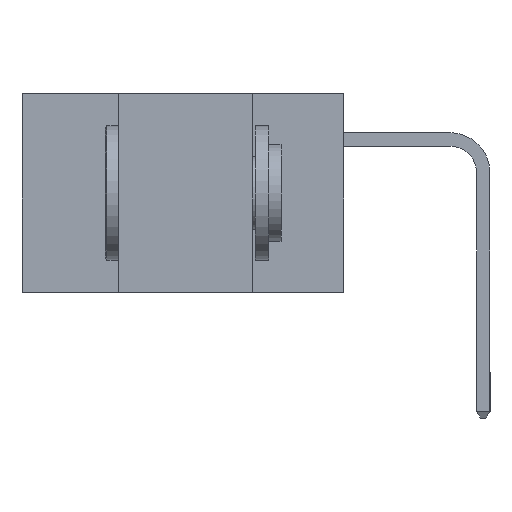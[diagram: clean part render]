
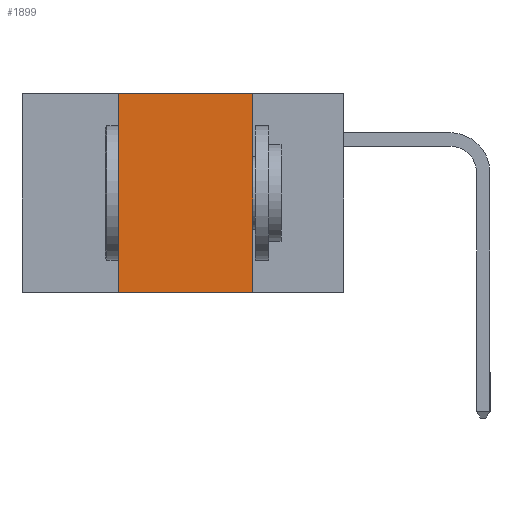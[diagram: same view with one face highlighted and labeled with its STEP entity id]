
A CAD part, left-side view. The second image highlights one B-rep face of the part: STEP entity #1899.
In plain terms, the highlighted planar face has unit normal (-1, 0, 0).
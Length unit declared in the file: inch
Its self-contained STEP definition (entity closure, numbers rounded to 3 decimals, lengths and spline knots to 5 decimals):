
#573 = LINE ( 'NONE', #4851, #6733 ) ;
#735 = CARTESIAN_POINT ( 'NONE',  ( 0., 0.42, 0. ) ) ;
#907 = DIRECTION ( 'NONE',  ( 0., -1., 0. ) ) ;
#1231 = CARTESIAN_POINT ( 'NONE',  ( 0., 0.17, -0.37 ) ) ;
#1440 = CARTESIAN_POINT ( 'NONE',  ( 0., 0.17, 0. ) ) ;
#1478 = LINE ( 'NONE', #7934, #7144 ) ;
#1799 = DIRECTION ( 'NONE',  ( 0., -1., 0. ) ) ;
#1844 = FACE_OUTER_BOUND ( 'NONE', #6764, .T. ) ;
#1899 = ADVANCED_FACE ( 'NONE', ( #1844 ), #7327, .F. ) ;
#2058 = AXIS2_PLACEMENT_3D ( 'NONE', #9640, #7390, #8138 ) ;
#2682 = EDGE_CURVE ( 'NONE', #4885, #6575, #4917, .T. ) ;
#3073 = ORIENTED_EDGE ( 'NONE', *, *, #7440, .F. ) ;
#3139 = VECTOR ( 'NONE', #6104, 39.37008 ) ;
#3254 = DIRECTION ( 'NONE',  ( 0., 0., 1. ) ) ;
#3515 = EDGE_CURVE ( 'NONE', #7877, #6575, #573, .T. ) ;
#4851 = CARTESIAN_POINT ( 'NONE',  ( 0., 0.6, -0.37 ) ) ;
#4885 = VERTEX_POINT ( 'NONE', #5595 ) ;
#4917 = LINE ( 'NONE', #1440, #3139 ) ;
#5148 = ORIENTED_EDGE ( 'NONE', *, *, #7636, .F. ) ;
#5404 = LINE ( 'NONE', #8667, #6499 ) ;
#5595 = CARTESIAN_POINT ( 'NONE',  ( 0., 0.17, 0. ) ) ;
#6104 = DIRECTION ( 'NONE',  ( 0., 0., -1. ) ) ;
#6499 = VECTOR ( 'NONE', #907, 39.37008 ) ;
#6575 = VERTEX_POINT ( 'NONE', #1231 ) ;
#6733 = VECTOR ( 'NONE', #1799, 39.37008 ) ;
#6764 = EDGE_LOOP ( 'NONE', ( #8663, #5148, #3073, #9223 ) ) ;
#7144 = VECTOR ( 'NONE', #3254, 39.37008 ) ;
#7327 = PLANE ( 'NONE',  #2058 ) ;
#7390 = DIRECTION ( 'NONE',  ( 1., 0., 0. ) ) ;
#7440 = EDGE_CURVE ( 'NONE', #7877, #9642, #1478, .T. ) ;
#7593 = CARTESIAN_POINT ( 'NONE',  ( 0., 0.42, -0.37 ) ) ;
#7636 = EDGE_CURVE ( 'NONE', #9642, #4885, #5404, .T. ) ;
#7877 = VERTEX_POINT ( 'NONE', #7593 ) ;
#7934 = CARTESIAN_POINT ( 'NONE',  ( 0., 0.42, 0. ) ) ;
#8138 = DIRECTION ( 'NONE',  ( 0., 0., -1. ) ) ;
#8663 = ORIENTED_EDGE ( 'NONE', *, *, #2682, .F. ) ;
#8667 = CARTESIAN_POINT ( 'NONE',  ( 0., 0.6, 0. ) ) ;
#9223 = ORIENTED_EDGE ( 'NONE', *, *, #3515, .T. ) ;
#9640 = CARTESIAN_POINT ( 'NONE',  ( 0., 0.6, 0. ) ) ;
#9642 = VERTEX_POINT ( 'NONE', #735 ) ;
